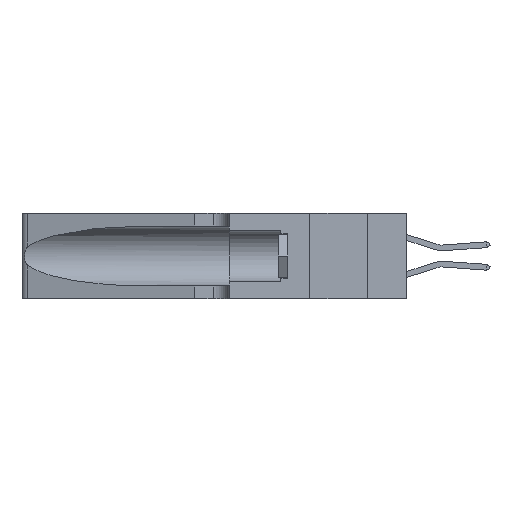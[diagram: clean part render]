
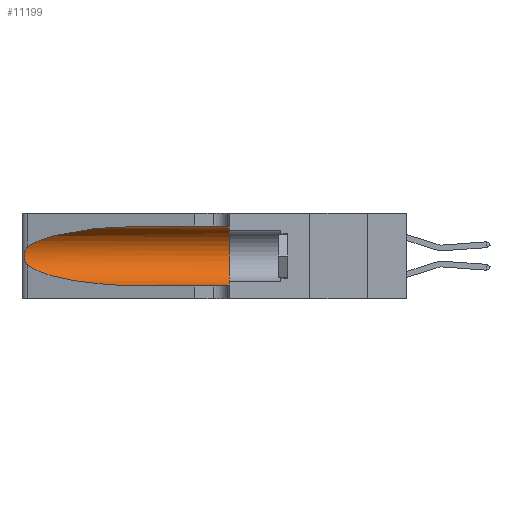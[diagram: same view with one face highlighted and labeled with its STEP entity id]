
A CAD part, left-side view. The second image highlights one B-rep face of the part: STEP entity #11199.
In plain terms, the highlighted cylindrical face has radius 3.308 mm (diameter 6.617 mm), a partial arc.
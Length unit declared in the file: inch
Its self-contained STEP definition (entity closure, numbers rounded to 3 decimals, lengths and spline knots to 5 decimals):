
#1011 = EDGE_CURVE ( 'NONE', #32748, #19344, #5332, .T. ) ;
#1516 = CARTESIAN_POINT ( 'NONE',  ( 0.25487, 1.22718, 0.14631 ) ) ;
#2004 = VERTEX_POINT ( 'NONE', #17517 ) ;
#2297 = CARTESIAN_POINT ( 'NONE',  ( 0.26017, 1.23833, 0.17102 ) ) ;
#2445 = CARTESIAN_POINT ( 'NONE',  ( 0.1305, 1.61858, 0.185 ) ) ;
#3376 = CARTESIAN_POINT ( 'NONE',  ( 0.1305, 0.35, 0.31525 ) ) ;
#4395 = VECTOR ( 'NONE', #25909, 39.37008 ) ;
#4703 = DIRECTION ( 'NONE',  ( 0., 1., 0. ) ) ;
#5314 = CARTESIAN_POINT ( 'NONE',  ( 0.25789, 1.23486, 0.15765 ) ) ;
#5332 = LINE ( 'NONE', #22336, #4395 ) ;
#5470 = DIRECTION ( 'NONE',  ( 0., 0., -1. ) ) ;
#5529 = EDGE_LOOP ( 'NONE', ( #18857, #26357, #34678, #36440, #6990, #22397 ) ) ;
#5958 = EDGE_CURVE ( 'NONE', #32748, #18946, #29823, .T. ) ;
#6990 = ORIENTED_EDGE ( 'NONE', *, *, #32295, .F. ) ;
#8179 = CARTESIAN_POINT ( 'NONE',  ( 0.25487, 1.22718, 0.22369 ) ) ;
#8307 = CARTESIAN_POINT ( 'NONE',  ( 0.25555, 1.22993, 0.14849 ) ) ;
#9585 = CARTESIAN_POINT ( 'NONE',  ( 0.1305, 0.72297, 0.31525 ) ) ;
#11199 = ADVANCED_FACE ( 'NONE', ( #15085 ), #29215, .F. ) ;
#12406 = EDGE_CURVE ( 'NONE', #13600, #2004, #16706, .T. ) ;
#12664 = VERTEX_POINT ( 'NONE', #23646 ) ;
#13600 = VERTEX_POINT ( 'NONE', #1516 ) ;
#13924 = B_SPLINE_CURVE_WITH_KNOTS ( 'NONE', 3,
 ( #8179, #25444, #31021, #14066, #33850, #16986, #36705, #19870, #2297, #22729, #5314, #25562, #8307, #28333 ),
 .UNSPECIFIED., .F., .F.,
 ( 4, 2, 2, 2, 2, 2, 4 ),
 ( 0., 0.00027, 0.00053, 0.00107, 0.0016, 0.00187, 0.00214 ),
 .UNSPECIFIED. ) ;
#14066 = CARTESIAN_POINT ( 'NONE',  ( 0.25787, 1.23484, 0.2124 ) ) ;
#14785 = CARTESIAN_POINT ( 'NONE',  ( 0.2373, 1.15595, 0.28018 ) ) ;
#15085 = FACE_OUTER_BOUND ( 'NONE', #5529, .T. ) ;
#16706 =( BOUNDED_CURVE ( )  B_SPLINE_CURVE ( 3, ( #19710, #33813, #36653, #19823 ),
 .UNSPECIFIED., .F., .F. ) 
 B_SPLINE_CURVE_WITH_KNOTS ( ( 4, 4 ),
 ( 3.44316, 4.71239 ),
 .UNSPECIFIED. ) 
 CURVE ( )  GEOMETRIC_REPRESENTATION_ITEM ( )  RATIONAL_B_SPLINE_CURVE ( ( 1., 0.87, 0.87, 1. ) ) 
 REPRESENTATION_ITEM ( '' )  );
#16986 = CARTESIAN_POINT ( 'NONE',  ( 0.26018, 1.23835, 0.19895 ) ) ;
#17517 = CARTESIAN_POINT ( 'NONE',  ( 0.1305, 0.72297, 0.05475 ) ) ;
#18148 = VECTOR ( 'NONE', #19711, 39.37008 ) ;
#18857 = ORIENTED_EDGE ( 'NONE', *, *, #5958, .T. ) ;
#18946 = VERTEX_POINT ( 'NONE', #19208 ) ;
#19208 = CARTESIAN_POINT ( 'NONE',  ( 0.25487, 1.22718, 0.22369 ) ) ;
#19344 = VERTEX_POINT ( 'NONE', #3376 ) ;
#19470 = AXIS2_PLACEMENT_3D ( 'NONE', #2445, #22859, #5470 ) ;
#19710 = CARTESIAN_POINT ( 'NONE',  ( 0.25487, 1.22718, 0.14631 ) ) ;
#19711 = DIRECTION ( 'NONE',  ( 0., -1., 0. ) ) ;
#19823 = CARTESIAN_POINT ( 'NONE',  ( 0.1305, 0.72297, 0.05475 ) ) ;
#19870 = CARTESIAN_POINT ( 'NONE',  ( 0.26075, 1.23896, 0.178 ) ) ;
#22130 = CARTESIAN_POINT ( 'NONE',  ( 0.1305, 0.35, 0.185 ) ) ;
#22336 = CARTESIAN_POINT ( 'NONE',  ( 0.1305, 1.61858, 0.31525 ) ) ;
#22397 = ORIENTED_EDGE ( 'NONE', *, *, #1011, .F. ) ;
#22729 = CARTESIAN_POINT ( 'NONE',  ( 0.25856, 1.23593, 0.16098 ) ) ;
#22859 = DIRECTION ( 'NONE',  ( 0., -1., 0. ) ) ;
#23646 = CARTESIAN_POINT ( 'NONE',  ( 0.1305, 0.35, 0.05475 ) ) ;
#24988 = DIRECTION ( 'NONE',  ( 0., 0., 1. ) ) ;
#25444 = CARTESIAN_POINT ( 'NONE',  ( 0.25555, 1.22994, 0.2215 ) ) ;
#25562 = CARTESIAN_POINT ( 'NONE',  ( 0.25639, 1.23186, 0.15144 ) ) ;
#25909 = DIRECTION ( 'NONE',  ( 0., -1., 0. ) ) ;
#26357 = ORIENTED_EDGE ( 'NONE', *, *, #28647, .T. ) ;
#26670 = CIRCLE ( 'NONE', #28691, 0.13025 ) ;
#28333 = CARTESIAN_POINT ( 'NONE',  ( 0.25487, 1.22718, 0.14631 ) ) ;
#28647 = EDGE_CURVE ( 'NONE', #18946, #13600, #13924, .T. ) ;
#28691 = AXIS2_PLACEMENT_3D ( 'NONE', #22130, #4703, #24988 ) ;
#28764 = CARTESIAN_POINT ( 'NONE',  ( 0.1305, 0.72297, 0.31525 ) ) ;
#29029 = EDGE_CURVE ( 'NONE', #2004, #12664, #32222, .T. ) ;
#29215 = CYLINDRICAL_SURFACE ( 'NONE', #19470, 0.13025 ) ;
#29823 =( BOUNDED_CURVE ( )  B_SPLINE_CURVE ( 3, ( #28764, #31704, #14785, #34555 ),
 .UNSPECIFIED., .F., .T. ) 
 B_SPLINE_CURVE_WITH_KNOTS ( ( 4, 4 ),
 ( 1.5708, 2.84003 ),
 .UNSPECIFIED. ) 
 CURVE ( )  GEOMETRIC_REPRESENTATION_ITEM ( )  RATIONAL_B_SPLINE_CURVE ( ( 1., 0.87, 0.87, 1. ) ) 
 REPRESENTATION_ITEM ( '' )  );
#31021 = CARTESIAN_POINT ( 'NONE',  ( 0.25639, 1.23184, 0.21858 ) ) ;
#31704 = CARTESIAN_POINT ( 'NONE',  ( 0.18966, 0.96281, 0.31525 ) ) ;
#32222 = LINE ( 'NONE', #33694, #18148 ) ;
#32295 = EDGE_CURVE ( 'NONE', #19344, #12664, #26670, .T. ) ;
#32748 = VERTEX_POINT ( 'NONE', #9585 ) ;
#33694 = CARTESIAN_POINT ( 'NONE',  ( 0.1305, 1.61858, 0.05475 ) ) ;
#33813 = CARTESIAN_POINT ( 'NONE',  ( 0.2373, 1.15595, 0.08982 ) ) ;
#33850 = CARTESIAN_POINT ( 'NONE',  ( 0.25854, 1.2359, 0.20912 ) ) ;
#34555 = CARTESIAN_POINT ( 'NONE',  ( 0.25487, 1.22718, 0.22369 ) ) ;
#34678 = ORIENTED_EDGE ( 'NONE', *, *, #12406, .T. ) ;
#36440 = ORIENTED_EDGE ( 'NONE', *, *, #29029, .T. ) ;
#36653 = CARTESIAN_POINT ( 'NONE',  ( 0.18966, 0.96281, 0.05475 ) ) ;
#36705 = CARTESIAN_POINT ( 'NONE',  ( 0.26075, 1.23896, 0.19203 ) ) ;
